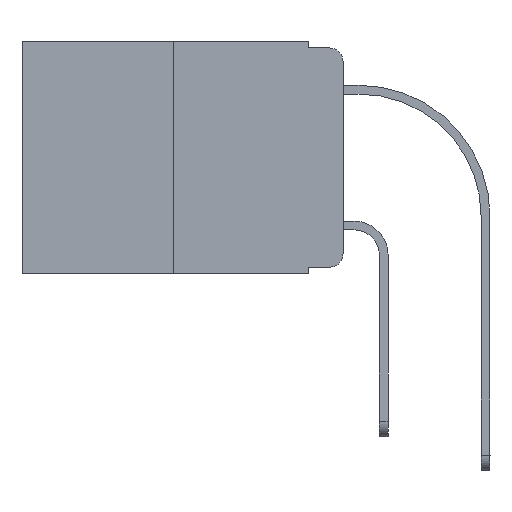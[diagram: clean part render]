
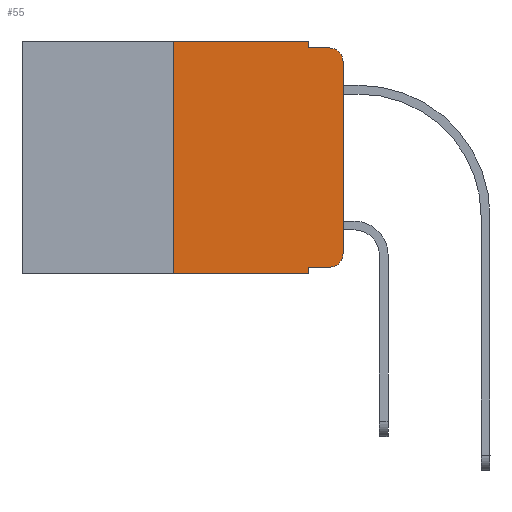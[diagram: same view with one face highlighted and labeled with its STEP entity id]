
A CAD part, left-side view. The second image highlights one B-rep face of the part: STEP entity #55.
In plain terms, the highlighted planar face has unit normal (-1, 0, 0).
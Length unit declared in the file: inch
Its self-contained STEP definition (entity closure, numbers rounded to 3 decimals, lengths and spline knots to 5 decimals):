
#55 = ADVANCED_FACE ( 'NONE', ( #9132 ), #1045, .F. ) ;
#161 = CARTESIAN_POINT ( 'NONE',  ( 0., 0.473, 0. ) ) ;
#214 = CIRCLE ( 'NONE', #1913, 0.02 ) ;
#339 = AXIS2_PLACEMENT_3D ( 'NONE', #161, #4864, #4630 ) ;
#455 = VERTEX_POINT ( 'NONE', #10059 ) ;
#510 = ORIENTED_EDGE ( 'NONE', *, *, #9802, .T. ) ;
#553 = ORIENTED_EDGE ( 'NONE', *, *, #5629, .F. ) ;
#655 = LINE ( 'NONE', #3298, #1689 ) ;
#1045 = PLANE ( 'NONE',  #339 ) ;
#1092 = LINE ( 'NONE', #5511, #8454 ) ;
#1162 = CARTESIAN_POINT ( 'NONE',  ( 0., 0., -0.313 ) ) ;
#1239 = CARTESIAN_POINT ( 'NONE',  ( 0., 0.051, -0.01 ) ) ;
#1476 = EDGE_CURVE ( 'NONE', #8431, #5666, #8424, .T. ) ;
#1536 = VECTOR ( 'NONE', #6150, 39.37008 ) ;
#1689 = VECTOR ( 'NONE', #3130, 39.37008 ) ;
#1748 = LINE ( 'NONE', #7934, #10374 ) ;
#1780 = EDGE_CURVE ( 'NONE', #3485, #4641, #11100, .T. ) ;
#1807 = CARTESIAN_POINT ( 'NONE',  ( 0., 0., 0. ) ) ;
#1875 = VECTOR ( 'NONE', #3000, 39.37008 ) ;
#1913 = AXIS2_PLACEMENT_3D ( 'NONE', #11461, #10575, #4212 ) ;
#2382 = CARTESIAN_POINT ( 'NONE',  ( 0., 0.02, -0.333 ) ) ;
#2434 = AXIS2_PLACEMENT_3D ( 'NONE', #3495, #7088, #10693 ) ;
#2818 = VECTOR ( 'NONE', #7425, 39.37008 ) ;
#2835 = CARTESIAN_POINT ( 'NONE',  ( 0., 0.051, -0.333 ) ) ;
#3000 = DIRECTION ( 'NONE',  ( 0., -1., 0. ) ) ;
#3003 = CARTESIAN_POINT ( 'NONE',  ( 0., 0.473, -0.343 ) ) ;
#3130 = DIRECTION ( 'NONE',  ( 0., 0., -1. ) ) ;
#3292 = VECTOR ( 'NONE', #9346, 39.37008 ) ;
#3298 = CARTESIAN_POINT ( 'NONE',  ( 0., 0.051, 0. ) ) ;
#3427 = VECTOR ( 'NONE', #4823, 39.37008 ) ;
#3485 = VERTEX_POINT ( 'NONE', #2835 ) ;
#3495 = CARTESIAN_POINT ( 'NONE',  ( 0., 0.02, -0.03 ) ) ;
#3572 = LINE ( 'NONE', #1807, #1536 ) ;
#3791 = VERTEX_POINT ( 'NONE', #5226 ) ;
#3830 = CARTESIAN_POINT ( 'NONE',  ( 0., 0.473, 0. ) ) ;
#4003 = ORIENTED_EDGE ( 'NONE', *, *, #5020, .F. ) ;
#4115 = ORIENTED_EDGE ( 'NONE', *, *, #8546, .F. ) ;
#4156 = VERTEX_POINT ( 'NONE', #11423 ) ;
#4212 = DIRECTION ( 'NONE',  ( 0., 0., -1. ) ) ;
#4232 = ORIENTED_EDGE ( 'NONE', *, *, #4346, .F. ) ;
#4346 = EDGE_CURVE ( 'NONE', #3485, #4156, #1092, .T. ) ;
#4630 = DIRECTION ( 'NONE',  ( 0., 0., -1. ) ) ;
#4641 = VERTEX_POINT ( 'NONE', #2382 ) ;
#4685 = CIRCLE ( 'NONE', #2434, 0.02 ) ;
#4733 = EDGE_CURVE ( 'NONE', #8305, #5666, #4685, .T. ) ;
#4823 = DIRECTION ( 'NONE',  ( 0., -1., 0. ) ) ;
#4838 = CARTESIAN_POINT ( 'NONE',  ( 0., 0.051, -0.333 ) ) ;
#4864 = DIRECTION ( 'NONE',  ( 1., 0., 0. ) ) ;
#5020 = EDGE_CURVE ( 'NONE', #455, #8431, #655, .T. ) ;
#5226 = CARTESIAN_POINT ( 'NONE',  ( 0., 0.25, -0.343 ) ) ;
#5333 = DIRECTION ( 'NONE',  ( 0., 0., 1. ) ) ;
#5511 = CARTESIAN_POINT ( 'NONE',  ( 0., 0.051, 0. ) ) ;
#5629 = EDGE_CURVE ( 'NONE', #3791, #6146, #1748, .T. ) ;
#5666 = VERTEX_POINT ( 'NONE', #10121 ) ;
#6146 = VERTEX_POINT ( 'NONE', #11588 ) ;
#6150 = DIRECTION ( 'NONE',  ( 0., 0., 1. ) ) ;
#7011 = CARTESIAN_POINT ( 'NONE',  ( 0., 0., -0.03 ) ) ;
#7088 = DIRECTION ( 'NONE',  ( -1., 0., 0. ) ) ;
#7273 = EDGE_CURVE ( 'NONE', #3791, #4156, #11150, .T. ) ;
#7296 = ORIENTED_EDGE ( 'NONE', *, *, #4733, .T. ) ;
#7425 = DIRECTION ( 'NONE',  ( 0., -1., 0. ) ) ;
#7431 = ORIENTED_EDGE ( 'NONE', *, *, #7805, .T. ) ;
#7805 = EDGE_CURVE ( 'NONE', #4641, #10651, #214, .T. ) ;
#7934 = CARTESIAN_POINT ( 'NONE',  ( 0., 0.25, 0. ) ) ;
#8127 = EDGE_LOOP ( 'NONE', ( #510, #7296, #8182, #4003, #4115, #553, #9151, #4232, #8315, #7431 ) ) ;
#8182 = ORIENTED_EDGE ( 'NONE', *, *, #1476, .F. ) ;
#8305 = VERTEX_POINT ( 'NONE', #7011 ) ;
#8313 = LINE ( 'NONE', #3830, #2818 ) ;
#8315 = ORIENTED_EDGE ( 'NONE', *, *, #1780, .T. ) ;
#8424 = LINE ( 'NONE', #9443, #1875 ) ;
#8431 = VERTEX_POINT ( 'NONE', #1239 ) ;
#8454 = VECTOR ( 'NONE', #10881, 39.37008 ) ;
#8546 = EDGE_CURVE ( 'NONE', #6146, #455, #8313, .T. ) ;
#9132 = FACE_OUTER_BOUND ( 'NONE', #8127, .T. ) ;
#9151 = ORIENTED_EDGE ( 'NONE', *, *, #7273, .T. ) ;
#9346 = DIRECTION ( 'NONE',  ( 0., -1., 0. ) ) ;
#9443 = CARTESIAN_POINT ( 'NONE',  ( 0., 0.051, -0.01 ) ) ;
#9802 = EDGE_CURVE ( 'NONE', #10651, #8305, #3572, .T. ) ;
#10059 = CARTESIAN_POINT ( 'NONE',  ( 0., 0.051, 0. ) ) ;
#10121 = CARTESIAN_POINT ( 'NONE',  ( 0., 0.02, -0.01 ) ) ;
#10374 = VECTOR ( 'NONE', #5333, 39.37008 ) ;
#10575 = DIRECTION ( 'NONE',  ( -1., 0., 0. ) ) ;
#10651 = VERTEX_POINT ( 'NONE', #1162 ) ;
#10693 = DIRECTION ( 'NONE',  ( 0., 0., -1. ) ) ;
#10881 = DIRECTION ( 'NONE',  ( 0., 0., -1. ) ) ;
#11100 = LINE ( 'NONE', #4838, #3292 ) ;
#11150 = LINE ( 'NONE', #3003, #3427 ) ;
#11423 = CARTESIAN_POINT ( 'NONE',  ( 0., 0.051, -0.343 ) ) ;
#11461 = CARTESIAN_POINT ( 'NONE',  ( 0., 0.02, -0.313 ) ) ;
#11588 = CARTESIAN_POINT ( 'NONE',  ( 0., 0.25, 0. ) ) ;
